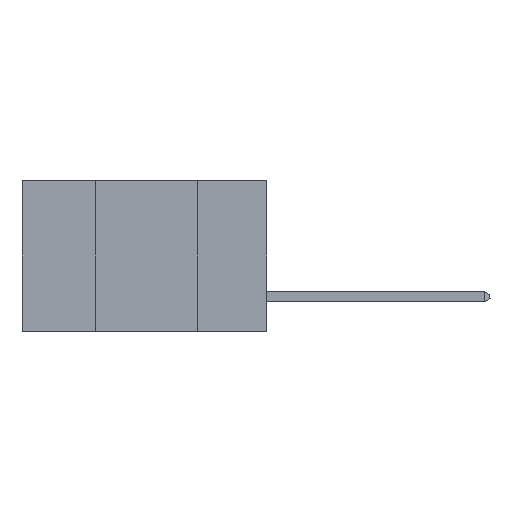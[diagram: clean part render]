
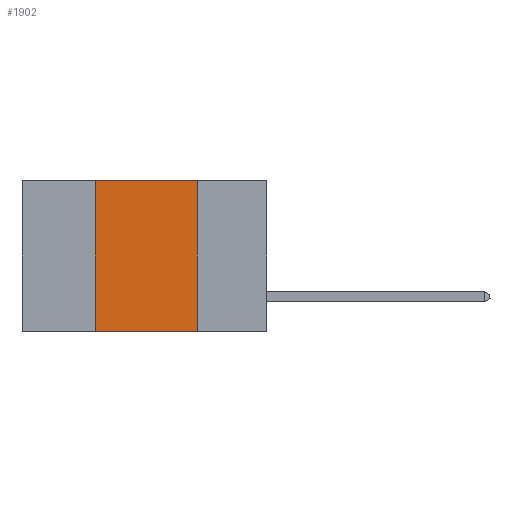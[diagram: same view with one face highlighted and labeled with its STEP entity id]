
A CAD part, left-side view. The second image highlights one B-rep face of the part: STEP entity #1902.
In plain terms, the highlighted planar face has unit normal (-1, 0, 0).
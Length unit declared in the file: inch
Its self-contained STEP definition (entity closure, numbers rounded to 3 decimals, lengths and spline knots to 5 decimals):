
#941 = DIRECTION ( 'NONE',  ( 0., 0., 1. ) ) ;
#1413 = CARTESIAN_POINT ( 'NONE',  ( 0., 0.17, 0. ) ) ;
#1428 = CARTESIAN_POINT ( 'NONE',  ( 0., 0.42, 0. ) ) ;
#1618 = CARTESIAN_POINT ( 'NONE',  ( 0., 0.6, 0. ) ) ;
#1902 = ADVANCED_FACE ( 'NONE', ( #19310 ), #20850, .F. ) ;
#2548 = AXIS2_PLACEMENT_3D ( 'NONE', #9933, #19065, #8392 ) ;
#2702 = ORIENTED_EDGE ( 'NONE', *, *, #14074, .T. ) ;
#3305 = VERTEX_POINT ( 'NONE', #1413 ) ;
#3374 = DIRECTION ( 'NONE',  ( 0., 0., -1. ) ) ;
#4902 = VECTOR ( 'NONE', #12759, 39.37008 ) ;
#5327 = VERTEX_POINT ( 'NONE', #19314 ) ;
#5627 = ORIENTED_EDGE ( 'NONE', *, *, #18200, .F. ) ;
#8392 = DIRECTION ( 'NONE',  ( 0., 0., -1. ) ) ;
#8494 = EDGE_CURVE ( 'NONE', #21352, #3305, #19915, .T. ) ;
#8655 = CARTESIAN_POINT ( 'NONE',  ( 0., 0.6, -0.37 ) ) ;
#8889 = LINE ( 'NONE', #16810, #22538 ) ;
#9008 = VERTEX_POINT ( 'NONE', #12558 ) ;
#9371 = LINE ( 'NONE', #8655, #4902 ) ;
#9933 = CARTESIAN_POINT ( 'NONE',  ( 0., 0.6, 0. ) ) ;
#9957 = EDGE_LOOP ( 'NONE', ( #5627, #15928, #12107, #2702 ) ) ;
#10443 = DIRECTION ( 'NONE',  ( 0., -1., 0. ) ) ;
#12065 = LINE ( 'NONE', #21249, #20118 ) ;
#12107 = ORIENTED_EDGE ( 'NONE', *, *, #13073, .F. ) ;
#12558 = CARTESIAN_POINT ( 'NONE',  ( 0., 0.42, -0.37 ) ) ;
#12759 = DIRECTION ( 'NONE',  ( 0., -1., 0. ) ) ;
#13073 = EDGE_CURVE ( 'NONE', #9008, #21352, #8889, .T. ) ;
#14074 = EDGE_CURVE ( 'NONE', #9008, #5327, #9371, .T. ) ;
#15928 = ORIENTED_EDGE ( 'NONE', *, *, #8494, .F. ) ;
#16810 = CARTESIAN_POINT ( 'NONE',  ( 0., 0.42, 0. ) ) ;
#18200 = EDGE_CURVE ( 'NONE', #3305, #5327, #12065, .T. ) ;
#19065 = DIRECTION ( 'NONE',  ( 1., 0., 0. ) ) ;
#19310 = FACE_OUTER_BOUND ( 'NONE', #9957, .T. ) ;
#19314 = CARTESIAN_POINT ( 'NONE',  ( 0., 0.17, -0.37 ) ) ;
#19915 = LINE ( 'NONE', #1618, #21288 ) ;
#20118 = VECTOR ( 'NONE', #3374, 39.37008 ) ;
#20850 = PLANE ( 'NONE',  #2548 ) ;
#21249 = CARTESIAN_POINT ( 'NONE',  ( 0., 0.17, 0. ) ) ;
#21288 = VECTOR ( 'NONE', #10443, 39.37008 ) ;
#21352 = VERTEX_POINT ( 'NONE', #1428 ) ;
#22538 = VECTOR ( 'NONE', #941, 39.37008 ) ;
